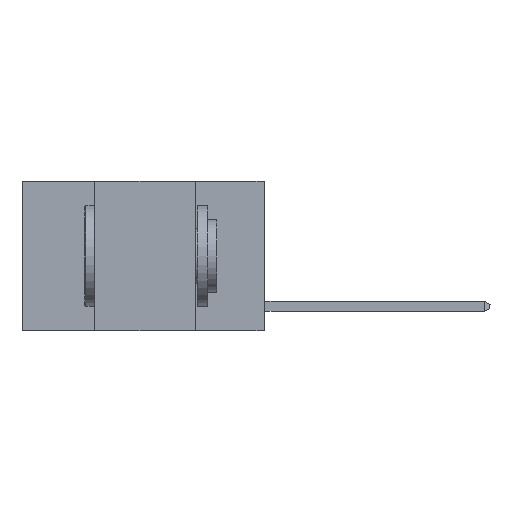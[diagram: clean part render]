
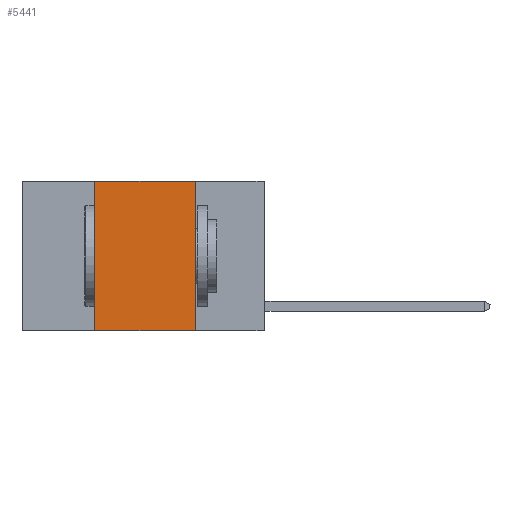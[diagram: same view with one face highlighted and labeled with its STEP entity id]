
A CAD part, left-side view. The second image highlights one B-rep face of the part: STEP entity #5441.
In plain terms, the highlighted planar face has unit normal (-1, 0, 0).
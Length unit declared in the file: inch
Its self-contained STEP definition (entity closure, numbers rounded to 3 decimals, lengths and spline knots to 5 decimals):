
#413 = LINE ( 'NONE', #4466, #10513 ) ;
#664 = PLANE ( 'NONE',  #18011 ) ;
#2481 = CARTESIAN_POINT ( 'NONE',  ( 0., 0.42, -0.37 ) ) ;
#2799 = DIRECTION ( 'NONE',  ( 0., 0., -1. ) ) ;
#3283 = DIRECTION ( 'NONE',  ( 0., 0., -1. ) ) ;
#3787 = ORIENTED_EDGE ( 'NONE', *, *, #22485, .F. ) ;
#4415 = ORIENTED_EDGE ( 'NONE', *, *, #23421, .F. ) ;
#4466 = CARTESIAN_POINT ( 'NONE',  ( 0., 0.6, 0. ) ) ;
#4913 = LINE ( 'NONE', #22096, #19650 ) ;
#5417 = ORIENTED_EDGE ( 'NONE', *, *, #12777, .F. ) ;
#5441 = ADVANCED_FACE ( 'NONE', ( #13114 ), #664, .F. ) ;
#7394 = EDGE_CURVE ( 'NONE', #13475, #14521, #4913, .T. ) ;
#8182 = DIRECTION ( 'NONE',  ( 0., 0., 1. ) ) ;
#10513 = VECTOR ( 'NONE', #16566, 39.37008 ) ;
#12777 = EDGE_CURVE ( 'NONE', #13475, #25050, #24632, .T. ) ;
#12849 = CARTESIAN_POINT ( 'NONE',  ( 0., 0.6, 0. ) ) ;
#13114 = FACE_OUTER_BOUND ( 'NONE', #14147, .T. ) ;
#13339 = CARTESIAN_POINT ( 'NONE',  ( 0., 0.17, 0. ) ) ;
#13475 = VERTEX_POINT ( 'NONE', #2481 ) ;
#13934 = VECTOR ( 'NONE', #3283, 39.37008 ) ;
#14147 = EDGE_LOOP ( 'NONE', ( #4415, #3787, #5417, #21060 ) ) ;
#14220 = CARTESIAN_POINT ( 'NONE',  ( 0., 0.42, 0. ) ) ;
#14521 = VERTEX_POINT ( 'NONE', #17528 ) ;
#14843 = DIRECTION ( 'NONE',  ( 1., 0., 0. ) ) ;
#15100 = VERTEX_POINT ( 'NONE', #21356 ) ;
#16566 = DIRECTION ( 'NONE',  ( 0., -1., 0. ) ) ;
#17528 = CARTESIAN_POINT ( 'NONE',  ( 0., 0.17, -0.37 ) ) ;
#18011 = AXIS2_PLACEMENT_3D ( 'NONE', #12849, #14843, #2799 ) ;
#19187 = LINE ( 'NONE', #13339, #13934 ) ;
#19650 = VECTOR ( 'NONE', #20170, 39.37008 ) ;
#20170 = DIRECTION ( 'NONE',  ( 0., -1., 0. ) ) ;
#20617 = VECTOR ( 'NONE', #8182, 39.37008 ) ;
#21060 = ORIENTED_EDGE ( 'NONE', *, *, #7394, .T. ) ;
#21356 = CARTESIAN_POINT ( 'NONE',  ( 0., 0.17, 0. ) ) ;
#22096 = CARTESIAN_POINT ( 'NONE',  ( 0., 0.6, -0.37 ) ) ;
#22240 = CARTESIAN_POINT ( 'NONE',  ( 0., 0.42, 0. ) ) ;
#22485 = EDGE_CURVE ( 'NONE', #25050, #15100, #413, .T. ) ;
#23421 = EDGE_CURVE ( 'NONE', #15100, #14521, #19187, .T. ) ;
#24632 = LINE ( 'NONE', #14220, #20617 ) ;
#25050 = VERTEX_POINT ( 'NONE', #22240 ) ;
